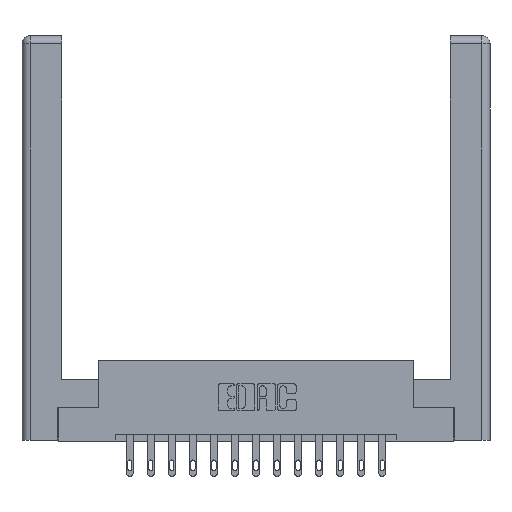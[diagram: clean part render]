
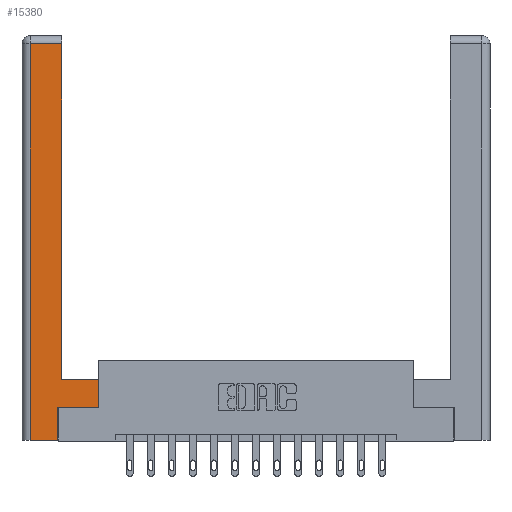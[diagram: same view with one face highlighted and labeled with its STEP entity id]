
A CAD part, top view. The second image highlights one B-rep face of the part: STEP entity #15380.
In plain terms, the highlighted planar face has unit normal (0, 0, 1).
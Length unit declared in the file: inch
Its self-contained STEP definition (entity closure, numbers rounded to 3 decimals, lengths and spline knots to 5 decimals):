
#70 = VERTEX_POINT ( 'NONE', #3621 ) ;
#226 = VECTOR ( 'NONE', #7894, 39.37008 ) ;
#466 = VERTEX_POINT ( 'NONE', #7100 ) ;
#1070 = EDGE_CURVE ( 'NONE', #466, #5218, #1759, .T. ) ;
#1480 = VERTEX_POINT ( 'NONE', #2061 ) ;
#1759 = LINE ( 'NONE', #11793, #11281 ) ;
#1995 = CARTESIAN_POINT ( 'NONE',  ( 0.0615, 2.94, 0. ) ) ;
#2061 = CARTESIAN_POINT ( 'NONE',  ( 0.565, 0.245, 0. ) ) ;
#2921 = VERTEX_POINT ( 'NONE', #10098 ) ;
#3029 = VERTEX_POINT ( 'NONE', #3552 ) ;
#3285 = EDGE_CURVE ( 'NONE', #5218, #3029, #12614, .T. ) ;
#3552 = CARTESIAN_POINT ( 'NONE',  ( 0.0615, 2.94, 0. ) ) ;
#3621 = CARTESIAN_POINT ( 'NONE',  ( 0.265, 0.245, 0. ) ) ;
#3898 = CARTESIAN_POINT ( 'NONE',  ( 0.0615, 0., 0. ) ) ;
#4111 = LINE ( 'NONE', #8217, #12407 ) ;
#4187 = CARTESIAN_POINT ( 'NONE',  ( 0.265, 0., 0. ) ) ;
#4364 = DIRECTION ( 'NONE',  ( 0., 1., 0. ) ) ;
#4544 = EDGE_LOOP ( 'NONE', ( #8717, #11111, #6625, #7020, #10675, #15825, #5567, #13930 ) ) ;
#4824 = VERTEX_POINT ( 'NONE', #11293 ) ;
#5218 = VERTEX_POINT ( 'NONE', #6159 ) ;
#5544 = VECTOR ( 'NONE', #15926, 39.37008 ) ;
#5567 = ORIENTED_EDGE ( 'NONE', *, *, #9751, .T. ) ;
#5636 = FACE_OUTER_BOUND ( 'NONE', #4544, .T. ) ;
#5801 = DIRECTION ( 'NONE',  ( -1., 0., 0. ) ) ;
#6159 = CARTESIAN_POINT ( 'NONE',  ( 0.295, 2.94, 0. ) ) ;
#6195 = LINE ( 'NONE', #6801, #226 ) ;
#6542 = DIRECTION ( 'NONE',  ( 1., 0., 0. ) ) ;
#6625 = ORIENTED_EDGE ( 'NONE', *, *, #15846, .T. ) ;
#6644 = PLANE ( 'NONE',  #11563 ) ;
#6801 = CARTESIAN_POINT ( 'NONE',  ( 0.265, 0.245, 0. ) ) ;
#7020 = ORIENTED_EDGE ( 'NONE', *, *, #15379, .T. ) ;
#7100 = CARTESIAN_POINT ( 'NONE',  ( 0.295, 0.45, 0. ) ) ;
#7435 = CARTESIAN_POINT ( 'NONE',  ( 0.0615, 0., 0. ) ) ;
#7476 = EDGE_CURVE ( 'NONE', #70, #1480, #8938, .T. ) ;
#7894 = DIRECTION ( 'NONE',  ( 0., 1., 0. ) ) ;
#8217 = CARTESIAN_POINT ( 'NONE',  ( 0.295, 0.45, 0. ) ) ;
#8647 = LINE ( 'NONE', #9004, #14923 ) ;
#8717 = ORIENTED_EDGE ( 'NONE', *, *, #1070, .T. ) ;
#8938 = LINE ( 'NONE', #13477, #5544 ) ;
#9004 = CARTESIAN_POINT ( 'NONE',  ( 0.565, 0.45, 0. ) ) ;
#9035 = VECTOR ( 'NONE', #6542, 39.37008 ) ;
#9138 = DIRECTION ( 'NONE',  ( 0., 0., -1. ) ) ;
#9598 = LINE ( 'NONE', #4187, #9035 ) ;
#9751 = EDGE_CURVE ( 'NONE', #1480, #2921, #8647, .T. ) ;
#10098 = CARTESIAN_POINT ( 'NONE',  ( 0.565, 0.45, 0. ) ) ;
#10430 = EDGE_CURVE ( 'NONE', #4824, #70, #6195, .T. ) ;
#10675 = ORIENTED_EDGE ( 'NONE', *, *, #10430, .T. ) ;
#11111 = ORIENTED_EDGE ( 'NONE', *, *, #3285, .T. ) ;
#11238 = VECTOR ( 'NONE', #5801, 39.37008 ) ;
#11281 = VECTOR ( 'NONE', #4364, 39.37008 ) ;
#11293 = CARTESIAN_POINT ( 'NONE',  ( 0.265, 0., 0. ) ) ;
#11563 = AXIS2_PLACEMENT_3D ( 'NONE', #12807, #9138, #14236 ) ;
#11793 = CARTESIAN_POINT ( 'NONE',  ( 0.295, 3., 0. ) ) ;
#12090 = DIRECTION ( 'NONE',  ( -1., 0., 0. ) ) ;
#12140 = VERTEX_POINT ( 'NONE', #7435 ) ;
#12407 = VECTOR ( 'NONE', #12090, 39.37008 ) ;
#12526 = VECTOR ( 'NONE', #12683, 39.37008 ) ;
#12614 = LINE ( 'NONE', #1995, #11238 ) ;
#12683 = DIRECTION ( 'NONE',  ( 0., -1., 0. ) ) ;
#12807 = CARTESIAN_POINT ( 'NONE',  ( 0., 0., 0. ) ) ;
#12945 = LINE ( 'NONE', #3898, #12526 ) ;
#13477 = CARTESIAN_POINT ( 'NONE',  ( 0.565, 0.245, 0. ) ) ;
#13817 = EDGE_CURVE ( 'NONE', #2921, #466, #4111, .T. ) ;
#13930 = ORIENTED_EDGE ( 'NONE', *, *, #13817, .T. ) ;
#14236 = DIRECTION ( 'NONE',  ( -1., 0., 0. ) ) ;
#14923 = VECTOR ( 'NONE', #15144, 39.37008 ) ;
#15144 = DIRECTION ( 'NONE',  ( 0., 1., 0. ) ) ;
#15379 = EDGE_CURVE ( 'NONE', #12140, #4824, #9598, .T. ) ;
#15380 = ADVANCED_FACE ( 'NONE', ( #5636 ), #6644, .F. ) ;
#15825 = ORIENTED_EDGE ( 'NONE', *, *, #7476, .T. ) ;
#15846 = EDGE_CURVE ( 'NONE', #3029, #12140, #12945, .T. ) ;
#15926 = DIRECTION ( 'NONE',  ( 1., 0., 0. ) ) ;
